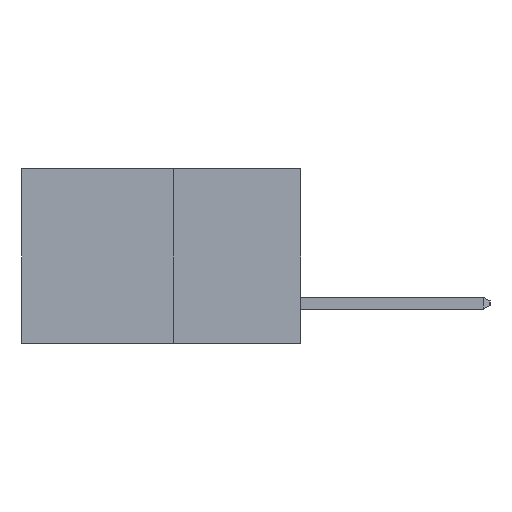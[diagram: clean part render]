
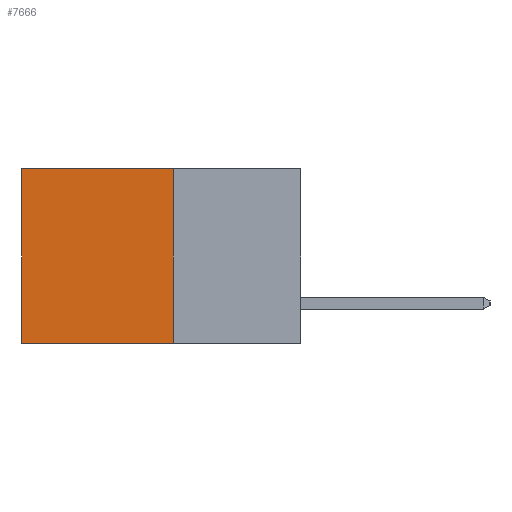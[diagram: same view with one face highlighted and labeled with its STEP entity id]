
A CAD part, left-side view. The second image highlights one B-rep face of the part: STEP entity #7666.
In plain terms, the highlighted planar face has unit normal (-1, 0, 0).
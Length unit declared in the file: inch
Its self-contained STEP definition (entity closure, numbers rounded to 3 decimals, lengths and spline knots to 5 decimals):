
#869 = CARTESIAN_POINT ( 'NONE',  ( 0.277, 0.59, 0. ) ) ;
#1040 = VERTEX_POINT ( 'NONE', #13118 ) ;
#1559 = VECTOR ( 'NONE', #13817, 39.37008 ) ;
#1766 = EDGE_CURVE ( 'NONE', #9982, #5571, #3572, .T. ) ;
#2327 = VECTOR ( 'NONE', #9563, 39.37008 ) ;
#2606 = VECTOR ( 'NONE', #12327, 39.37008 ) ;
#3572 = LINE ( 'NONE', #13846, #1559 ) ;
#4919 = EDGE_CURVE ( 'NONE', #1040, #11510, #8409, .T. ) ;
#5005 = EDGE_LOOP ( 'NONE', ( #6371, #11119, #6659, #6616 ) ) ;
#5571 = VERTEX_POINT ( 'NONE', #6689 ) ;
#5927 = VECTOR ( 'NONE', #12602, 39.37008 ) ;
#6100 = AXIS2_PLACEMENT_3D ( 'NONE', #10573, #10426, #10422 ) ;
#6371 = ORIENTED_EDGE ( 'NONE', *, *, #12401, .T. ) ;
#6616 = ORIENTED_EDGE ( 'NONE', *, *, #4919, .T. ) ;
#6659 = ORIENTED_EDGE ( 'NONE', *, *, #6819, .F. ) ;
#6689 = CARTESIAN_POINT ( 'NONE',  ( 0.277, 0.59, -0.37 ) ) ;
#6819 = EDGE_CURVE ( 'NONE', #1040, #9982, #12044, .T. ) ;
#6993 = FACE_OUTER_BOUND ( 'NONE', #5005, .T. ) ;
#7666 = ADVANCED_FACE ( 'NONE', ( #6993 ), #11030, .F. ) ;
#8409 = LINE ( 'NONE', #12042, #2606 ) ;
#9563 = DIRECTION ( 'NONE',  ( 0., 0., -1. ) ) ;
#9908 = CARTESIAN_POINT ( 'NONE',  ( 0.277, 0.27, -0.37 ) ) ;
#9982 = VERTEX_POINT ( 'NONE', #9908 ) ;
#10422 = DIRECTION ( 'NONE',  ( 0., 0., -1. ) ) ;
#10426 = DIRECTION ( 'NONE',  ( 1., 0., 0. ) ) ;
#10573 = CARTESIAN_POINT ( 'NONE',  ( 0.277, 0.27, -0.37 ) ) ;
#11030 = PLANE ( 'NONE',  #6100 ) ;
#11119 = ORIENTED_EDGE ( 'NONE', *, *, #1766, .F. ) ;
#11510 = VERTEX_POINT ( 'NONE', #869 ) ;
#11542 = LINE ( 'NONE', #14098, #2327 ) ;
#12042 = CARTESIAN_POINT ( 'NONE',  ( 0.277, 0.27, 0. ) ) ;
#12044 = LINE ( 'NONE', #12651, #5927 ) ;
#12327 = DIRECTION ( 'NONE',  ( 0., 1., 0. ) ) ;
#12401 = EDGE_CURVE ( 'NONE', #11510, #5571, #11542, .T. ) ;
#12602 = DIRECTION ( 'NONE',  ( 0., 0., -1. ) ) ;
#12651 = CARTESIAN_POINT ( 'NONE',  ( 0.277, 0.27, -0.37 ) ) ;
#13118 = CARTESIAN_POINT ( 'NONE',  ( 0.277, 0.27, 0. ) ) ;
#13817 = DIRECTION ( 'NONE',  ( 0., 1., 0. ) ) ;
#13846 = CARTESIAN_POINT ( 'NONE',  ( 0.277, 0.27, -0.37 ) ) ;
#14098 = CARTESIAN_POINT ( 'NONE',  ( 0.277, 0.59, -0.37 ) ) ;
